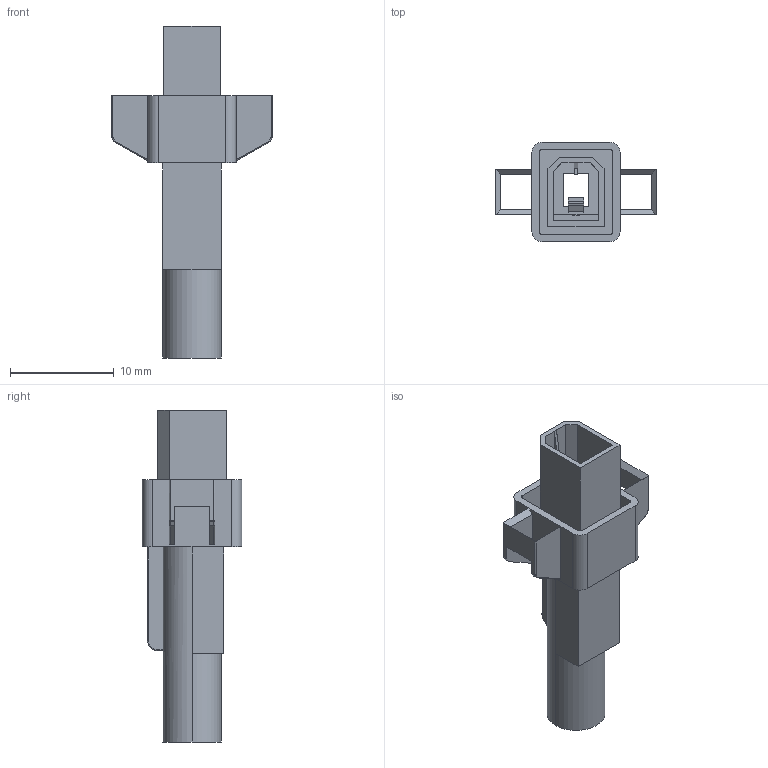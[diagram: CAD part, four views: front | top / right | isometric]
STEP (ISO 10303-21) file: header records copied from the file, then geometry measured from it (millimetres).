
FILE_DESCRIPTION (( 'STEP AP214' ), '1' );
FILE_NAME ('567-001-000-310.STEP', '2020-07-27T19:36:59', ( '' ), ( '' ), 'SwSTEP 2.0', 'SolidWorks 2020', '' );
FILE_SCHEMA (( 'AUTOMOTIVE_DESIGN' ));
Length unit declared in the file: millimetre
Products named in the file (1): 567-001-000-310
Bounding box: 15.5 x 9.6 x 32 mm (x, y, z)
Volume: 642.2 mm3; surface area: 1976.2 mm2
Topology: 1 solids, 1 shells, 163 faces, 446 edges, 274 vertices
Faces by surface type: plane 116, cylinder 37, sphere 8, torus 2
Entity records: 5082 total; most frequent: CARTESIAN_POINT 948, ORIENTED_EDGE 876, DIRECTION 836, EDGE_CURVE 438, VECTOR 336, LINE 336, VERTEX_POINT 274, AXIS2_PLACEMENT_3D 250
